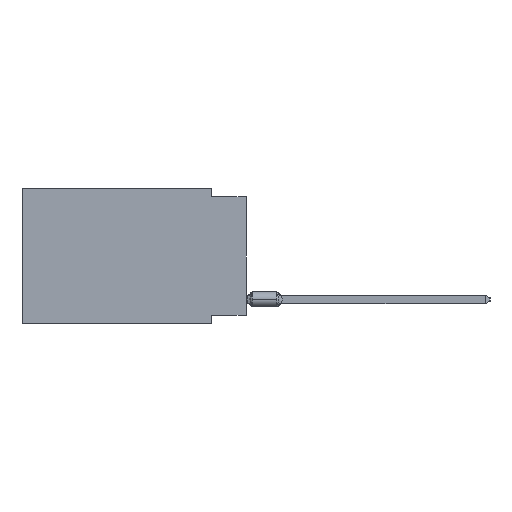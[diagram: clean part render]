
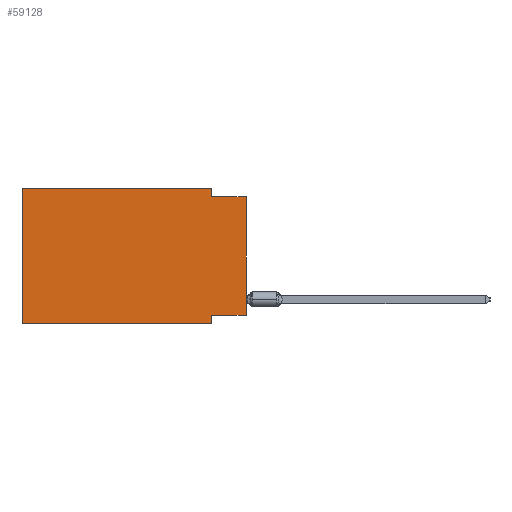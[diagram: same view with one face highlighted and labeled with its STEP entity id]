
A CAD part, left-side view. The second image highlights one B-rep face of the part: STEP entity #59128.
In plain terms, the highlighted planar face has unit normal (-1, 0, 0).
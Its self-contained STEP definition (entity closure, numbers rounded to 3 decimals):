
#390 = ORIENTED_EDGE ( 'NONE', *, *, #76402, .F. ) ;
#2674 = EDGE_CURVE ( 'NONE', #20053, #85332, #86423, .T. ) ;
#6408 = VECTOR ( 'NONE', #42834, 1000. ) ;
#7026 = DIRECTION ( 'NONE',  ( 0., 0., 1. ) ) ;
#7056 = EDGE_CURVE ( 'NONE', #39428, #57844, #48999, .T. ) ;
#8591 = EDGE_CURVE ( 'NONE', #47981, #85332, #18516, .T. ) ;
#9241 = CARTESIAN_POINT ( 'NONE',  ( 0., 0., -9.271 ) ) ;
#9349 = DIRECTION ( 'NONE',  ( 0., 0., -1. ) ) ;
#9957 = FACE_OUTER_BOUND ( 'NONE', #26438, .T. ) ;
#12407 = ORIENTED_EDGE ( 'NONE', *, *, #76723, .F. ) ;
#14083 = CARTESIAN_POINT ( 'NONE',  ( 0., 2.54, 0. ) ) ;
#14173 = CARTESIAN_POINT ( 'NONE',  ( 0., 16.383, 0. ) ) ;
#15026 = VECTOR ( 'NONE', #24272, 1000. ) ;
#16086 = CARTESIAN_POINT ( 'NONE',  ( 0., 16.383, 0. ) ) ;
#16727 = CARTESIAN_POINT ( 'NONE',  ( 0., 2.54, 0. ) ) ;
#17022 = ORIENTED_EDGE ( 'NONE', *, *, #54968, .T. ) ;
#18051 = VECTOR ( 'NONE', #9349, 1000. ) ;
#18282 = CARTESIAN_POINT ( 'NONE',  ( 0., 16.383, -9.906 ) ) ;
#18516 = LINE ( 'NONE', #32089, #34631 ) ;
#20053 = VERTEX_POINT ( 'NONE', #9241 ) ;
#24272 = DIRECTION ( 'NONE',  ( 0., 1., 0. ) ) ;
#26438 = EDGE_LOOP ( 'NONE', ( #41511, #49264, #53949, #64716, #390, #17022, #12407, #35667 ) ) ;
#29988 = LINE ( 'NONE', #65058, #15026 ) ;
#30629 = CARTESIAN_POINT ( 'NONE',  ( 0., 2.54, -9.906 ) ) ;
#32089 = CARTESIAN_POINT ( 'NONE',  ( 0., 0., -0.635 ) ) ;
#33778 = CARTESIAN_POINT ( 'NONE',  ( 0., 16.383, -9.906 ) ) ;
#34631 = VECTOR ( 'NONE', #38247, 1000. ) ;
#35667 = ORIENTED_EDGE ( 'NONE', *, *, #45095, .F. ) ;
#38247 = DIRECTION ( 'NONE',  ( 0., -1., 0. ) ) ;
#38659 = VERTEX_POINT ( 'NONE', #18282 ) ;
#39428 = VERTEX_POINT ( 'NONE', #14173 ) ;
#41511 = ORIENTED_EDGE ( 'NONE', *, *, #2674, .T. ) ;
#42834 = DIRECTION ( 'NONE',  ( 0., -1., 0. ) ) ;
#43100 = LINE ( 'NONE', #56679, #18051 ) ;
#45091 = CARTESIAN_POINT ( 'NONE',  ( 0., 2.54, -0.635 ) ) ;
#45095 = EDGE_CURVE ( 'NONE', #20053, #59092, #29988, .T. ) ;
#46928 = CARTESIAN_POINT ( 'NONE',  ( 0., 0., 0. ) ) ;
#47895 = VERTEX_POINT ( 'NONE', #30629 ) ;
#47981 = VERTEX_POINT ( 'NONE', #45091 ) ;
#48877 = VECTOR ( 'NONE', #67917, 1000. ) ;
#48999 = LINE ( 'NONE', #16086, #6408 ) ;
#49017 = DIRECTION ( 'NONE',  ( 0., 0., -1. ) ) ;
#49264 = ORIENTED_EDGE ( 'NONE', *, *, #8591, .F. ) ;
#53501 = VECTOR ( 'NONE', #60546, 1000. ) ;
#53949 = ORIENTED_EDGE ( 'NONE', *, *, #63530, .F. ) ;
#54968 = EDGE_CURVE ( 'NONE', #38659, #47895, #67132, .T. ) ;
#56679 = CARTESIAN_POINT ( 'NONE',  ( 0., 2.54, -9.906 ) ) ;
#57844 = VERTEX_POINT ( 'NONE', #14083 ) ;
#59092 = VERTEX_POINT ( 'NONE', #86785 ) ;
#59128 = ADVANCED_FACE ( 'NONE', ( #9957 ), #69195, .F. ) ;
#60546 = DIRECTION ( 'NONE',  ( 0., -1., 0. ) ) ;
#60893 = LINE ( 'NONE', #74499, #48877 ) ;
#62800 = DIRECTION ( 'NONE',  ( 0., 0., -1. ) ) ;
#63530 = EDGE_CURVE ( 'NONE', #57844, #47981, #68524, .T. ) ;
#64716 = ORIENTED_EDGE ( 'NONE', *, *, #7056, .F. ) ;
#65058 = CARTESIAN_POINT ( 'NONE',  ( 0., 0., -9.271 ) ) ;
#67132 = LINE ( 'NONE', #33778, #53501 ) ;
#67917 = DIRECTION ( 'NONE',  ( 0., 0., 1. ) ) ;
#68524 = LINE ( 'NONE', #16727, #80935 ) ;
#69195 = PLANE ( 'NONE',  #72138 ) ;
#70446 = CARTESIAN_POINT ( 'NONE',  ( 0., 0., -0.635 ) ) ;
#72138 = AXIS2_PLACEMENT_3D ( 'NONE', #76644, #75357, #49017 ) ;
#74499 = CARTESIAN_POINT ( 'NONE',  ( 0., 16.383, 0. ) ) ;
#75357 = DIRECTION ( 'NONE',  ( 1., 0., 0. ) ) ;
#76402 = EDGE_CURVE ( 'NONE', #38659, #39428, #60893, .T. ) ;
#76644 = CARTESIAN_POINT ( 'NONE',  ( 0., 16.383, 0. ) ) ;
#76723 = EDGE_CURVE ( 'NONE', #59092, #47895, #43100, .T. ) ;
#80935 = VECTOR ( 'NONE', #62800, 1000. ) ;
#85332 = VERTEX_POINT ( 'NONE', #70446 ) ;
#85804 = VECTOR ( 'NONE', #7026, 1000. ) ;
#86423 = LINE ( 'NONE', #46928, #85804 ) ;
#86785 = CARTESIAN_POINT ( 'NONE',  ( 0., 2.54, -9.271 ) ) ;
